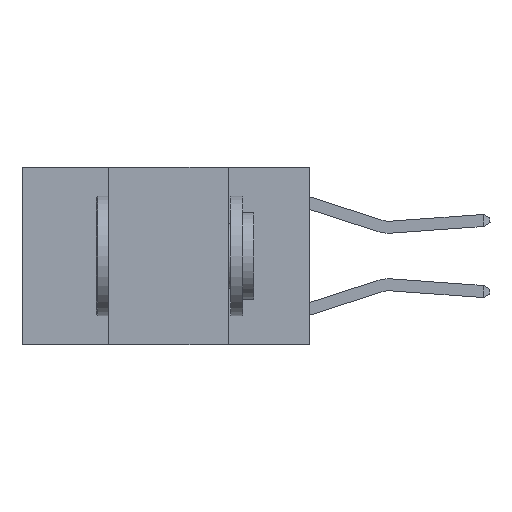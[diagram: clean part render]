
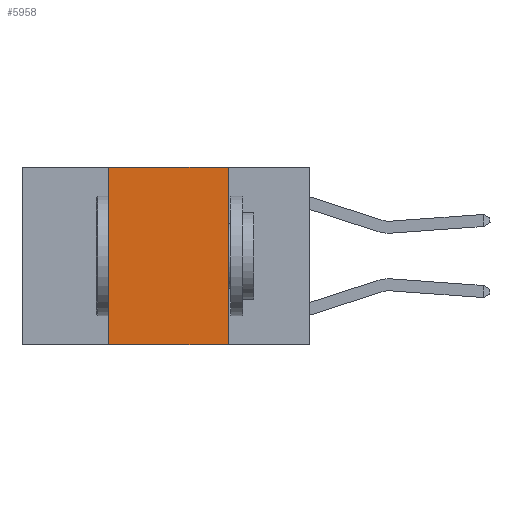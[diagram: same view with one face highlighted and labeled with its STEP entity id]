
A CAD part, left-side view. The second image highlights one B-rep face of the part: STEP entity #5958.
In plain terms, the highlighted planar face has unit normal (-1, 0, 0).
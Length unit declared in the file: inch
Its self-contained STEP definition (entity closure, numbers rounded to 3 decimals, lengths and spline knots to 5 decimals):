
#534 = VECTOR ( 'NONE', #7852, 39.37008 ) ;
#588 = VERTEX_POINT ( 'NONE', #6072 ) ;
#857 = CARTESIAN_POINT ( 'NONE',  ( 0., 0.17, 0. ) ) ;
#865 = CARTESIAN_POINT ( 'NONE',  ( 0., 0.17, 0. ) ) ;
#995 = VERTEX_POINT ( 'NONE', #3846 ) ;
#1045 = PLANE ( 'NONE',  #4491 ) ;
#1360 = ORIENTED_EDGE ( 'NONE', *, *, #5579, .F. ) ;
#1510 = ORIENTED_EDGE ( 'NONE', *, *, #9594, .F. ) ;
#1672 = ORIENTED_EDGE ( 'NONE', *, *, #5066, .F. ) ;
#1692 = EDGE_CURVE ( 'NONE', #995, #588, #7127, .T. ) ;
#1757 = ORIENTED_EDGE ( 'NONE', *, *, #1692, .T. ) ;
#1900 = DIRECTION ( 'NONE',  ( 0., 0., -1. ) ) ;
#2211 = VERTEX_POINT ( 'NONE', #857 ) ;
#2713 = DIRECTION ( 'NONE',  ( 0., 0., 1. ) ) ;
#3456 = LINE ( 'NONE', #865, #7516 ) ;
#3775 = VECTOR ( 'NONE', #8547, 39.37008 ) ;
#3846 = CARTESIAN_POINT ( 'NONE',  ( 0., 0.42, -0.37 ) ) ;
#3989 = VECTOR ( 'NONE', #2713, 39.37008 ) ;
#4400 = CARTESIAN_POINT ( 'NONE',  ( 0., 0.6, 0. ) ) ;
#4491 = AXIS2_PLACEMENT_3D ( 'NONE', #4400, #6832, #1900 ) ;
#5066 = EDGE_CURVE ( 'NONE', #995, #9777, #6152, .T. ) ;
#5150 = CARTESIAN_POINT ( 'NONE',  ( 0., 0.42, 0. ) ) ;
#5579 = EDGE_CURVE ( 'NONE', #2211, #588, #3456, .T. ) ;
#5958 = ADVANCED_FACE ( 'NONE', ( #8984 ), #1045, .F. ) ;
#6072 = CARTESIAN_POINT ( 'NONE',  ( 0., 0.17, -0.37 ) ) ;
#6152 = LINE ( 'NONE', #5150, #3989 ) ;
#6199 = LINE ( 'NONE', #9332, #3775 ) ;
#6662 = DIRECTION ( 'NONE',  ( 0., 0., -1. ) ) ;
#6832 = DIRECTION ( 'NONE',  ( 1., 0., 0. ) ) ;
#7127 = LINE ( 'NONE', #8036, #534 ) ;
#7516 = VECTOR ( 'NONE', #6662, 39.37008 ) ;
#7852 = DIRECTION ( 'NONE',  ( 0., -1., 0. ) ) ;
#8036 = CARTESIAN_POINT ( 'NONE',  ( 0., 0.6, -0.37 ) ) ;
#8547 = DIRECTION ( 'NONE',  ( 0., -1., 0. ) ) ;
#8759 = CARTESIAN_POINT ( 'NONE',  ( 0., 0.42, 0. ) ) ;
#8984 = FACE_OUTER_BOUND ( 'NONE', #9506, .T. ) ;
#9332 = CARTESIAN_POINT ( 'NONE',  ( 0., 0.6, 0. ) ) ;
#9506 = EDGE_LOOP ( 'NONE', ( #1360, #1510, #1672, #1757 ) ) ;
#9594 = EDGE_CURVE ( 'NONE', #9777, #2211, #6199, .T. ) ;
#9777 = VERTEX_POINT ( 'NONE', #8759 ) ;
